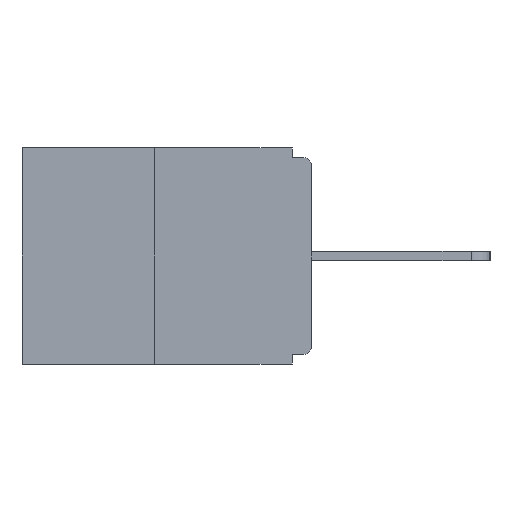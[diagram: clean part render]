
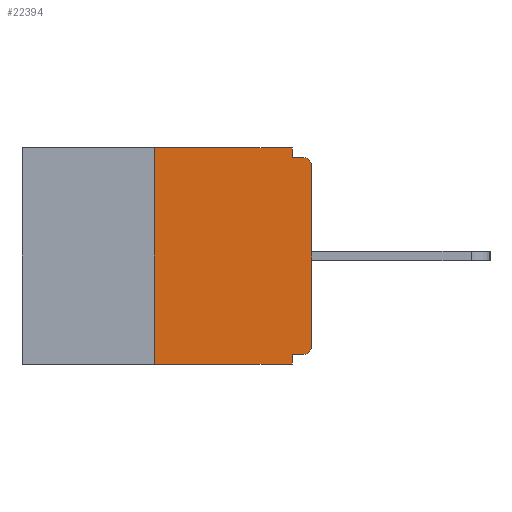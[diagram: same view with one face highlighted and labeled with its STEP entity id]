
A CAD part, left-side view. The second image highlights one B-rep face of the part: STEP entity #22394.
In plain terms, the highlighted planar face has unit normal (-1, 0, 0).
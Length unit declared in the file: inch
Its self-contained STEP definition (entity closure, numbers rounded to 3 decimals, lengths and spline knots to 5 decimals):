
#680 = DIRECTION ( 'NONE',  ( 0., 0., -1. ) ) ;
#1137 = VERTEX_POINT ( 'NONE', #1984 ) ;
#1592 = AXIS2_PLACEMENT_3D ( 'NONE', #21476, #10597, #23287 ) ;
#1622 = VERTEX_POINT ( 'NONE', #19623 ) ;
#1732 = LINE ( 'NONE', #19818, #20597 ) ;
#1826 = VERTEX_POINT ( 'NONE', #16368 ) ;
#1984 = CARTESIAN_POINT ( 'NONE',  ( 0., 0., -0.03 ) ) ;
#2255 = LINE ( 'NONE', #3882, #11446 ) ;
#2628 = CARTESIAN_POINT ( 'NONE',  ( 0., 0., -0.328 ) ) ;
#2668 = EDGE_LOOP ( 'NONE', ( #22742, #13707, #9958, #19643, #12252, #17686, #22476, #8525, #9127, #18811 ) ) ;
#3231 = CARTESIAN_POINT ( 'NONE',  ( 0., 0.031, 0. ) ) ;
#3278 = EDGE_CURVE ( 'NONE', #19846, #15486, #7889, .T. ) ;
#3488 = AXIS2_PLACEMENT_3D ( 'NONE', #19394, #10307, #23019 ) ;
#3882 = CARTESIAN_POINT ( 'NONE',  ( 0., 0.25, 0. ) ) ;
#3957 = DIRECTION ( 'NONE',  ( 0., 0., 1. ) ) ;
#4205 = CARTESIAN_POINT ( 'NONE',  ( 0., 0.031, -0.328 ) ) ;
#4431 = LINE ( 'NONE', #20177, #8132 ) ;
#5404 = EDGE_CURVE ( 'NONE', #1826, #17614, #13543, .T. ) ;
#5646 = CARTESIAN_POINT ( 'NONE',  ( 0., 0.031, -0.343 ) ) ;
#5753 = EDGE_CURVE ( 'NONE', #17614, #1137, #6081, .T. ) ;
#6081 = LINE ( 'NONE', #20163, #15234 ) ;
#6339 = FACE_OUTER_BOUND ( 'NONE', #2668, .T. ) ;
#6588 = EDGE_CURVE ( 'NONE', #10351, #1622, #2255, .T. ) ;
#6662 = PLANE ( 'NONE',  #3488 ) ;
#7210 = EDGE_CURVE ( 'NONE', #1622, #8773, #22245, .T. ) ;
#7739 = VECTOR ( 'NONE', #680, 39.37008 ) ;
#7889 = LINE ( 'NONE', #19641, #17071 ) ;
#8132 = VECTOR ( 'NONE', #22000, 39.37008 ) ;
#8525 = ORIENTED_EDGE ( 'NONE', *, *, #10178, .T. ) ;
#8773 = VERTEX_POINT ( 'NONE', #3231 ) ;
#8978 = VERTEX_POINT ( 'NONE', #5646 ) ;
#9127 = ORIENTED_EDGE ( 'NONE', *, *, #3278, .F. ) ;
#9629 = DIRECTION ( 'NONE',  ( 0., -1., 0. ) ) ;
#9958 = ORIENTED_EDGE ( 'NONE', *, *, #10887, .T. ) ;
#10178 = EDGE_CURVE ( 'NONE', #1137, #15486, #17262, .T. ) ;
#10307 = DIRECTION ( 'NONE',  ( 1., 0., 0. ) ) ;
#10351 = VERTEX_POINT ( 'NONE', #14784 ) ;
#10597 = DIRECTION ( 'NONE',  ( -1., 0., 0. ) ) ;
#10658 = LINE ( 'NONE', #2628, #19783 ) ;
#10729 = DIRECTION ( 'NONE',  ( 0., -1., 0. ) ) ;
#10887 = EDGE_CURVE ( 'NONE', #10351, #8978, #1732, .T. ) ;
#11236 = EDGE_CURVE ( 'NONE', #8773, #19846, #17480, .T. ) ;
#11446 = VECTOR ( 'NONE', #3957, 39.37008 ) ;
#11778 = CARTESIAN_POINT ( 'NONE',  ( 0., 0.031, 0. ) ) ;
#12252 = ORIENTED_EDGE ( 'NONE', *, *, #15017, .F. ) ;
#12415 = CARTESIAN_POINT ( 'NONE',  ( 0., 0.031, -0.015 ) ) ;
#13543 = CIRCLE ( 'NONE', #22031, 0.015 ) ;
#13707 = ORIENTED_EDGE ( 'NONE', *, *, #6588, .F. ) ;
#14215 = CARTESIAN_POINT ( 'NONE',  ( 0., 0., -0.313 ) ) ;
#14784 = CARTESIAN_POINT ( 'NONE',  ( 0., 0.25, -0.343 ) ) ;
#15017 = EDGE_CURVE ( 'NONE', #1826, #17315, #10658, .T. ) ;
#15234 = VECTOR ( 'NONE', #20190, 39.37008 ) ;
#15486 = VERTEX_POINT ( 'NONE', #16852 ) ;
#16368 = CARTESIAN_POINT ( 'NONE',  ( 0., 0.015, -0.328 ) ) ;
#16852 = CARTESIAN_POINT ( 'NONE',  ( 0., 0.015, -0.015 ) ) ;
#17071 = VECTOR ( 'NONE', #10729, 39.37008 ) ;
#17262 = CIRCLE ( 'NONE', #1592, 0.015 ) ;
#17274 = DIRECTION ( 'NONE',  ( 0., 1., 0. ) ) ;
#17315 = VERTEX_POINT ( 'NONE', #4205 ) ;
#17451 = VECTOR ( 'NONE', #9629, 39.37008 ) ;
#17480 = LINE ( 'NONE', #11778, #7739 ) ;
#17614 = VERTEX_POINT ( 'NONE', #14215 ) ;
#17686 = ORIENTED_EDGE ( 'NONE', *, *, #5404, .T. ) ;
#18724 = CARTESIAN_POINT ( 'NONE',  ( 0., 0.46, 0. ) ) ;
#18811 = ORIENTED_EDGE ( 'NONE', *, *, #11236, .F. ) ;
#19394 = CARTESIAN_POINT ( 'NONE',  ( 0., 0.46, 0. ) ) ;
#19623 = CARTESIAN_POINT ( 'NONE',  ( 0., 0.25, 0. ) ) ;
#19641 = CARTESIAN_POINT ( 'NONE',  ( 0., 0., -0.015 ) ) ;
#19643 = ORIENTED_EDGE ( 'NONE', *, *, #20052, .F. ) ;
#19645 = CARTESIAN_POINT ( 'NONE',  ( 0., 0.015, -0.313 ) ) ;
#19763 = DIRECTION ( 'NONE',  ( 0., 0., -1. ) ) ;
#19783 = VECTOR ( 'NONE', #17274, 39.37008 ) ;
#19787 = DIRECTION ( 'NONE',  ( -1., 0., 0. ) ) ;
#19818 = CARTESIAN_POINT ( 'NONE',  ( 0., 0.46, -0.343 ) ) ;
#19846 = VERTEX_POINT ( 'NONE', #12415 ) ;
#20052 = EDGE_CURVE ( 'NONE', #17315, #8978, #4431, .T. ) ;
#20163 = CARTESIAN_POINT ( 'NONE',  ( 0., 0., 0. ) ) ;
#20177 = CARTESIAN_POINT ( 'NONE',  ( 0., 0.031, -0.343 ) ) ;
#20190 = DIRECTION ( 'NONE',  ( 0., 0., 1. ) ) ;
#20597 = VECTOR ( 'NONE', #23419, 39.37008 ) ;
#21476 = CARTESIAN_POINT ( 'NONE',  ( 0., 0.015, -0.03 ) ) ;
#22000 = DIRECTION ( 'NONE',  ( 0., 0., -1. ) ) ;
#22031 = AXIS2_PLACEMENT_3D ( 'NONE', #19645, #19787, #19763 ) ;
#22245 = LINE ( 'NONE', #18724, #17451 ) ;
#22394 = ADVANCED_FACE ( 'NONE', ( #6339 ), #6662, .F. ) ;
#22476 = ORIENTED_EDGE ( 'NONE', *, *, #5753, .T. ) ;
#22742 = ORIENTED_EDGE ( 'NONE', *, *, #7210, .F. ) ;
#23019 = DIRECTION ( 'NONE',  ( 0., 0., -1. ) ) ;
#23287 = DIRECTION ( 'NONE',  ( 0., 0., -1. ) ) ;
#23419 = DIRECTION ( 'NONE',  ( 0., -1., 0. ) ) ;
